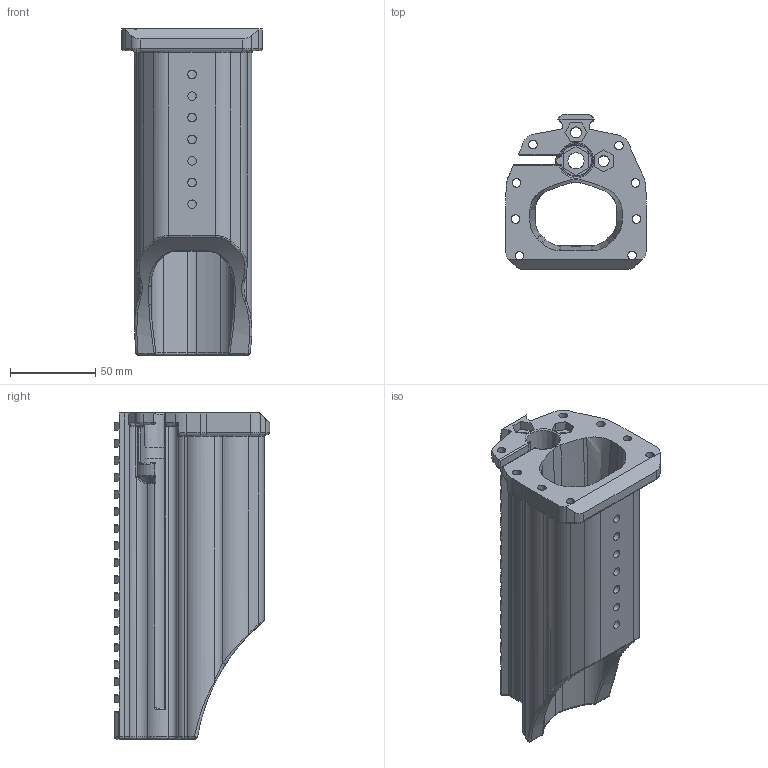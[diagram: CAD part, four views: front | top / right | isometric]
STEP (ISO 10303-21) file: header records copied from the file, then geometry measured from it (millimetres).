
FILE_DESCRIPTION(/* description */ (''),/* implementation_level */ '2;1');
FILE_NAME(/* name */ 'Handguard-Cocking Tube Rev4.stp',/* time_stamp */ '2021-10-03T20:57:34-05:00',/* author */ ('johne'),/* organization */ (''),/* preprocessor_version */ 'ST-DEVELOPER v18.1',/* originating_system */ 'Autodesk Inventor 2020',/* authorisation */ '');
FILE_SCHEMA (('AUTOMOTIVE_DESIGN { 1 0 10303 214 3 1 1 }'));
Length unit declared in the file: inch
Products named in the file (1): Handguard-Cocking Tube
Bounding box: 82.76 x 91.19 x 191.39 mm (x, y, z)
Volume: 393214.3 mm3; surface area: 99737.1 mm2
Topology: 1 solids, 1 shells, 517 faces, 1364 edges, 839 vertices
Faces by surface type: plane 247, cylinder 117, bspline 77, torus 59, sphere 11, cone 6
Full cylindrical faces by diameter (mm): 5 x15, 6.477 x2, 9.525 x1
Entity records: 18043 total; most frequent: CARTESIAN_POINT 5381, ORIENTED_EDGE 2710, DIRECTION 2539, EDGE_CURVE 1355, AXIS2_PLACEMENT_3D 861, VERTEX_POINT 839, LINE 817, VECTOR 817
